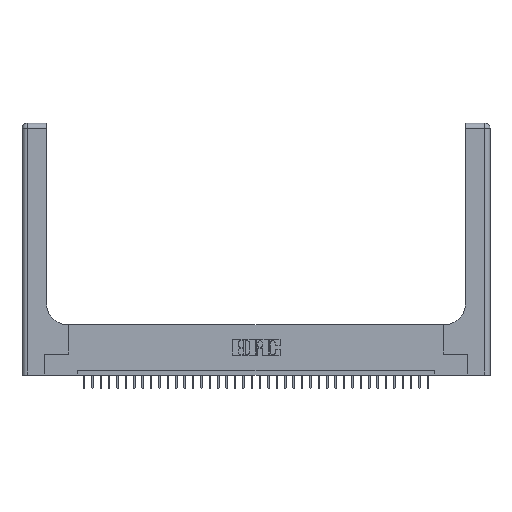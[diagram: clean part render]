
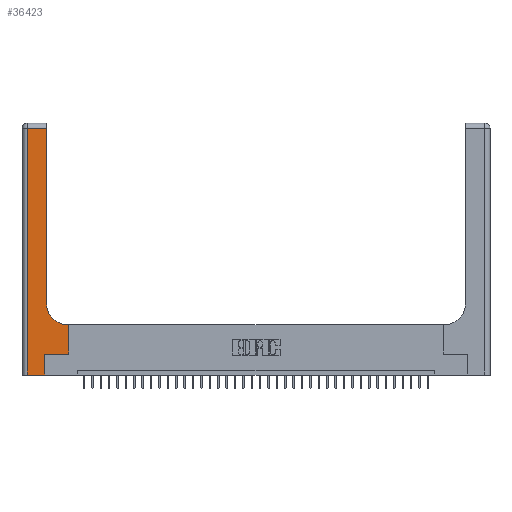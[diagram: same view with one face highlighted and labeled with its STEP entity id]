
A CAD part, top view. The second image highlights one B-rep face of the part: STEP entity #36423.
In plain terms, the highlighted planar face has unit normal (0, 0, 1).
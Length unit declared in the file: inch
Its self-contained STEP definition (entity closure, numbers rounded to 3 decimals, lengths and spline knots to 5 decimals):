
#641 = EDGE_CURVE ( 'NONE', #32177, #11425, #29401, .T. ) ;
#864 = ORIENTED_EDGE ( 'NONE', *, *, #3394, .T. ) ;
#1007 = VECTOR ( 'NONE', #33262, 39.37008 ) ;
#1053 = VERTEX_POINT ( 'NONE', #5483 ) ;
#1475 = DIRECTION ( 'NONE',  ( 0., 0., -1. ) ) ;
#1623 = DIRECTION ( 'NONE',  ( 1., 0., 0. ) ) ;
#1695 = LINE ( 'NONE', #1703, #7912 ) ;
#1703 = CARTESIAN_POINT ( 'NONE',  ( 0.5585, 0.25, 0.37 ) ) ;
#3394 = EDGE_CURVE ( 'NONE', #17503, #30499, #9152, .T. ) ;
#3445 = CARTESIAN_POINT ( 'NONE',  ( 0.269, 0., 0.37 ) ) ;
#4397 = LINE ( 'NONE', #16872, #8895 ) ;
#4879 = AXIS2_PLACEMENT_3D ( 'NONE', #18873, #1475, #21385 ) ;
#5483 = CARTESIAN_POINT ( 'NONE',  ( 0.06, 0., 0.37 ) ) ;
#5633 = ORIENTED_EDGE ( 'NONE', *, *, #10332, .T. ) ;
#6708 = EDGE_CURVE ( 'NONE', #8816, #32177, #10063, .T. ) ;
#6739 = EDGE_CURVE ( 'NONE', #16214, #31733, #10522, .T. ) ;
#6749 = CARTESIAN_POINT ( 'NONE',  ( 0.2915, 3., 0.37 ) ) ;
#7363 = ORIENTED_EDGE ( 'NONE', *, *, #28906, .T. ) ;
#7912 = VECTOR ( 'NONE', #24713, 39.37008 ) ;
#8597 = CARTESIAN_POINT ( 'NONE',  ( 0.269, 0.25, 0.37 ) ) ;
#8816 = VERTEX_POINT ( 'NONE', #9309 ) ;
#8895 = VECTOR ( 'NONE', #25451, 39.37008 ) ;
#9152 = LINE ( 'NONE', #15298, #28313 ) ;
#9309 = CARTESIAN_POINT ( 'NONE',  ( 0.5585, 0.6, 0.37 ) ) ;
#9541 = EDGE_CURVE ( 'NONE', #11425, #16214, #26300, .T. ) ;
#10063 = LINE ( 'NONE', #32716, #18068 ) ;
#10332 = EDGE_CURVE ( 'NONE', #1053, #13618, #4397, .T. ) ;
#10522 = LINE ( 'NONE', #23987, #19429 ) ;
#11425 = VERTEX_POINT ( 'NONE', #11551 ) ;
#11551 = CARTESIAN_POINT ( 'NONE',  ( 0.2915, 0.85, 0.37 ) ) ;
#12048 = DIRECTION ( 'NONE',  ( 0., 1., 0. ) ) ;
#13368 = VECTOR ( 'NONE', #17970, 39.37008 ) ;
#13516 = CARTESIAN_POINT ( 'NONE',  ( 0.5415, 0.85, 0.37 ) ) ;
#13618 = VERTEX_POINT ( 'NONE', #3445 ) ;
#13984 = CARTESIAN_POINT ( 'NONE',  ( 0.5415, 0.6, 0.37 ) ) ;
#15298 = CARTESIAN_POINT ( 'NONE',  ( 0.269, 0.25, 0.37 ) ) ;
#16214 = VERTEX_POINT ( 'NONE', #23308 ) ;
#16568 = CARTESIAN_POINT ( 'NONE',  ( 0.06, 3., 0.37 ) ) ;
#16872 = CARTESIAN_POINT ( 'NONE',  ( 0., 0., 0.37 ) ) ;
#17008 = EDGE_CURVE ( 'NONE', #31733, #1053, #24627, .T. ) ;
#17503 = VERTEX_POINT ( 'NONE', #8597 ) ;
#17970 = DIRECTION ( 'NONE',  ( 0., 1., 0. ) ) ;
#18068 = VECTOR ( 'NONE', #35577, 39.37008 ) ;
#18873 = CARTESIAN_POINT ( 'NONE',  ( 0., 3., 0.37 ) ) ;
#19429 = VECTOR ( 'NONE', #32217, 39.37008 ) ;
#20000 = EDGE_LOOP ( 'NONE', ( #25528, #29067, #26969, #5633, #7363, #864, #20423, #29935, #23352 ) ) ;
#20423 = ORIENTED_EDGE ( 'NONE', *, *, #27456, .T. ) ;
#21385 = DIRECTION ( 'NONE',  ( -1., 0., 0. ) ) ;
#23308 = CARTESIAN_POINT ( 'NONE',  ( 0.2915, 2.94, 0.37 ) ) ;
#23352 = ORIENTED_EDGE ( 'NONE', *, *, #641, .T. ) ;
#23987 = CARTESIAN_POINT ( 'NONE',  ( 0., 2.94, 0.37 ) ) ;
#24481 = DIRECTION ( 'NONE',  ( 1., 0., 0. ) ) ;
#24627 = LINE ( 'NONE', #16568, #1007 ) ;
#24713 = DIRECTION ( 'NONE',  ( 0., 1., 0. ) ) ;
#24880 = AXIS2_PLACEMENT_3D ( 'NONE', #13516, #36044, #24481 ) ;
#25451 = DIRECTION ( 'NONE',  ( 1., 0., 0. ) ) ;
#25528 = ORIENTED_EDGE ( 'NONE', *, *, #9541, .T. ) ;
#26300 = LINE ( 'NONE', #6749, #13368 ) ;
#26969 = ORIENTED_EDGE ( 'NONE', *, *, #17008, .T. ) ;
#27433 = VECTOR ( 'NONE', #12048, 39.37008 ) ;
#27456 = EDGE_CURVE ( 'NONE', #30499, #8816, #1695, .T. ) ;
#28313 = VECTOR ( 'NONE', #1623, 39.37008 ) ;
#28906 = EDGE_CURVE ( 'NONE', #13618, #17503, #34971, .T. ) ;
#29067 = ORIENTED_EDGE ( 'NONE', *, *, #6739, .T. ) ;
#29213 = CARTESIAN_POINT ( 'NONE',  ( 0.06, 2.94, 0.37 ) ) ;
#29382 = CARTESIAN_POINT ( 'NONE',  ( 0.269, 0., 0.37 ) ) ;
#29401 = CIRCLE ( 'NONE', #24880, 0.25 ) ;
#29935 = ORIENTED_EDGE ( 'NONE', *, *, #6708, .T. ) ;
#30499 = VERTEX_POINT ( 'NONE', #33959 ) ;
#31236 = FACE_OUTER_BOUND ( 'NONE', #20000, .T. ) ;
#31733 = VERTEX_POINT ( 'NONE', #29213 ) ;
#32177 = VERTEX_POINT ( 'NONE', #13984 ) ;
#32217 = DIRECTION ( 'NONE',  ( -1., 0., 0. ) ) ;
#32716 = CARTESIAN_POINT ( 'NONE',  ( 0.2915, 0.6, 0.37 ) ) ;
#33262 = DIRECTION ( 'NONE',  ( 0., -1., 0. ) ) ;
#33959 = CARTESIAN_POINT ( 'NONE',  ( 0.5585, 0.25, 0.37 ) ) ;
#34971 = LINE ( 'NONE', #29382, #27433 ) ;
#35565 = PLANE ( 'NONE',  #4879 ) ;
#35577 = DIRECTION ( 'NONE',  ( -1., 0., 0. ) ) ;
#36044 = DIRECTION ( 'NONE',  ( 0., 0., -1. ) ) ;
#36423 = ADVANCED_FACE ( 'NONE', ( #31236 ), #35565, .F. ) ;
